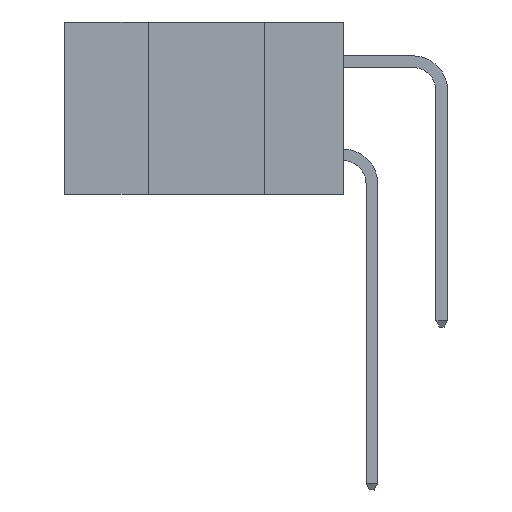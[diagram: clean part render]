
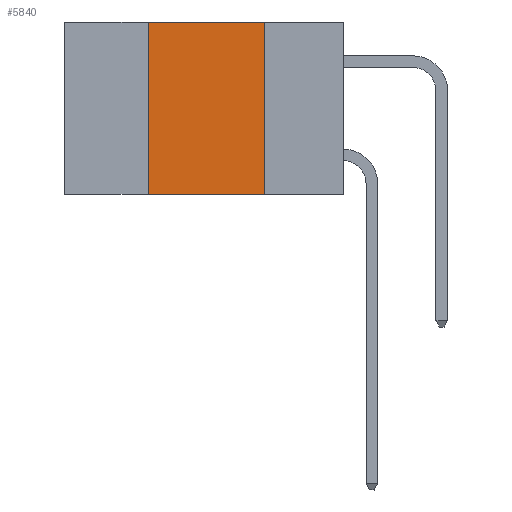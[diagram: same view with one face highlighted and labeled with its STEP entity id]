
A CAD part, left-side view. The second image highlights one B-rep face of the part: STEP entity #5840.
In plain terms, the highlighted planar face has unit normal (-1, 0, 0).
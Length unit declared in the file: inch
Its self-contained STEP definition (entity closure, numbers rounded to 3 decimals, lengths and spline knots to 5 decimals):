
#1472 = LINE ( 'NONE', #14834, #5720 ) ;
#2014 = EDGE_CURVE ( 'NONE', #11691, #11542, #6276, .T. ) ;
#2691 = VERTEX_POINT ( 'NONE', #5403 ) ;
#2692 = VECTOR ( 'NONE', #6410, 39.37008 ) ;
#2891 = ORIENTED_EDGE ( 'NONE', *, *, #10974, .F. ) ;
#3153 = LINE ( 'NONE', #16611, #6061 ) ;
#3223 = DIRECTION ( 'NONE',  ( 1., 0., 0. ) ) ;
#3664 = DIRECTION ( 'NONE',  ( 0., 0., 1. ) ) ;
#3920 = CARTESIAN_POINT ( 'NONE',  ( 0., 0.42, 0. ) ) ;
#4243 = CARTESIAN_POINT ( 'NONE',  ( 0., 0.17, -0.37 ) ) ;
#4983 = CARTESIAN_POINT ( 'NONE',  ( 0., 0.6, -0.37 ) ) ;
#5403 = CARTESIAN_POINT ( 'NONE',  ( 0., 0.42, -0.37 ) ) ;
#5720 = VECTOR ( 'NONE', #3664, 39.37008 ) ;
#5786 = VERTEX_POINT ( 'NONE', #4243 ) ;
#5840 = ADVANCED_FACE ( 'NONE', ( #11612 ), #13721, .F. ) ;
#5962 = ORIENTED_EDGE ( 'NONE', *, *, #2014, .F. ) ;
#5977 = EDGE_CURVE ( 'NONE', #2691, #11691, #1472, .T. ) ;
#6061 = VECTOR ( 'NONE', #10904, 39.37008 ) ;
#6085 = ORIENTED_EDGE ( 'NONE', *, *, #5977, .F. ) ;
#6276 = LINE ( 'NONE', #11713, #17145 ) ;
#6410 = DIRECTION ( 'NONE',  ( 0., -1., 0. ) ) ;
#7502 = ORIENTED_EDGE ( 'NONE', *, *, #15395, .T. ) ;
#9255 = CARTESIAN_POINT ( 'NONE',  ( 0., 0.17, 0. ) ) ;
#10153 = LINE ( 'NONE', #4983, #2692 ) ;
#10904 = DIRECTION ( 'NONE',  ( 0., 0., -1. ) ) ;
#10974 = EDGE_CURVE ( 'NONE', #11542, #5786, #3153, .T. ) ;
#11529 = DIRECTION ( 'NONE',  ( 0., 0., -1. ) ) ;
#11542 = VERTEX_POINT ( 'NONE', #9255 ) ;
#11612 = FACE_OUTER_BOUND ( 'NONE', #14524, .T. ) ;
#11691 = VERTEX_POINT ( 'NONE', #3920 ) ;
#11713 = CARTESIAN_POINT ( 'NONE',  ( 0., 0.6, 0. ) ) ;
#11875 = DIRECTION ( 'NONE',  ( 0., -1., 0. ) ) ;
#12718 = CARTESIAN_POINT ( 'NONE',  ( 0., 0.6, 0. ) ) ;
#13721 = PLANE ( 'NONE',  #16254 ) ;
#14524 = EDGE_LOOP ( 'NONE', ( #2891, #5962, #6085, #7502 ) ) ;
#14834 = CARTESIAN_POINT ( 'NONE',  ( 0., 0.42, 0. ) ) ;
#15395 = EDGE_CURVE ( 'NONE', #2691, #5786, #10153, .T. ) ;
#16254 = AXIS2_PLACEMENT_3D ( 'NONE', #12718, #3223, #11529 ) ;
#16611 = CARTESIAN_POINT ( 'NONE',  ( 0., 0.17, 0. ) ) ;
#17145 = VECTOR ( 'NONE', #11875, 39.37008 ) ;
